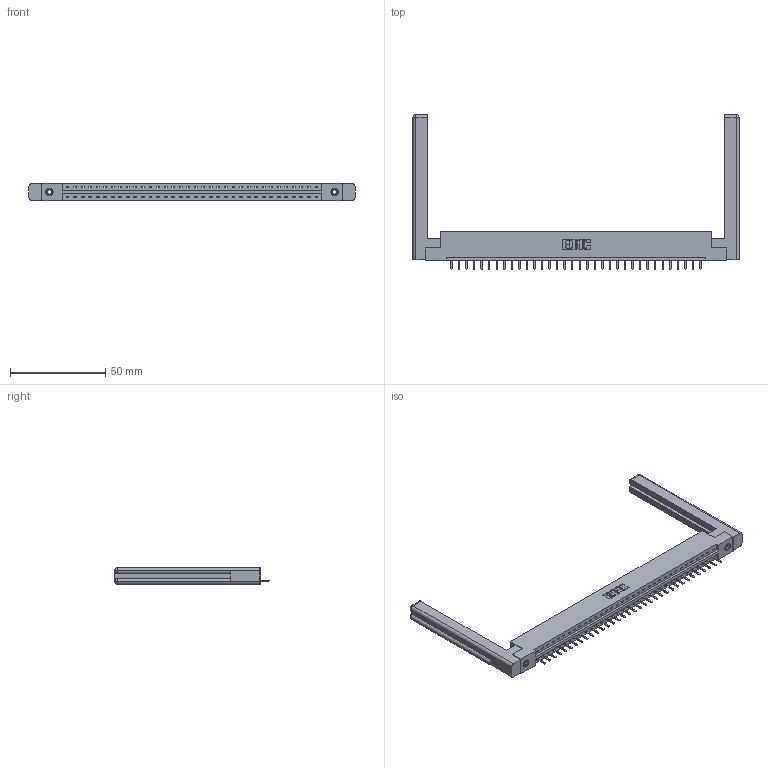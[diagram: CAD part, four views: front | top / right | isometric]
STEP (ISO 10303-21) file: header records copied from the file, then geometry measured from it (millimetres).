
FILE_DESCRIPTION (( 'STEP AP203' ), '1' );
FILE_NAME ('387-034-520-158.STEP', '2019-10-04T10:48:46', ( '' ), ( '' ), 'SwSTEP 2.0', 'SolidWorks 2016', '' );
FILE_SCHEMA (( 'CONFIG_CONTROL_DESIGN' ));
Length unit declared in the file: inch
Products named in the file (5): 307-220-058; 345-292-001_345-293-120; 345-250-001_345-250-001-102; 337 Part_Flush Mounting Lugs - 0.156 Dia-TI; 387-034-520-158
Assembly tree (39 placements, depth 2):
  387-034-520-158
    337 Part_Flush Mounting Lugs - 0.156 Dia-TI
    345-292-001_345-293-120  x34
    345-250-001_345-250-001-102  x2
    307-220-058  x2
Bounding box: 171.35 x 81.11 x 9.4 mm (x, y, z)
Volume: 24773 mm3; surface area: 23014.8 mm2
Topology: 39 solids, 39 shells, 2500 faces, 7329 edges, 4782 vertices
Faces by surface type: plane 1786, cylinder 690, cone 12, torus 12
Entity records: 29056 total; most frequent: CARTESIAN_POINT 5071, ORIENTED_EDGE 4968, DIRECTION 4292, EDGE_CURVE 2484, VECTOR 2304, LINE 2304, VERTEX_POINT 1646, AXIS2_PLACEMENT_3D 994
